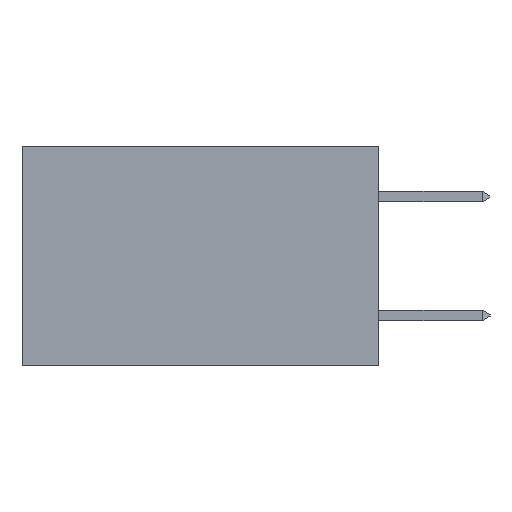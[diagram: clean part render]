
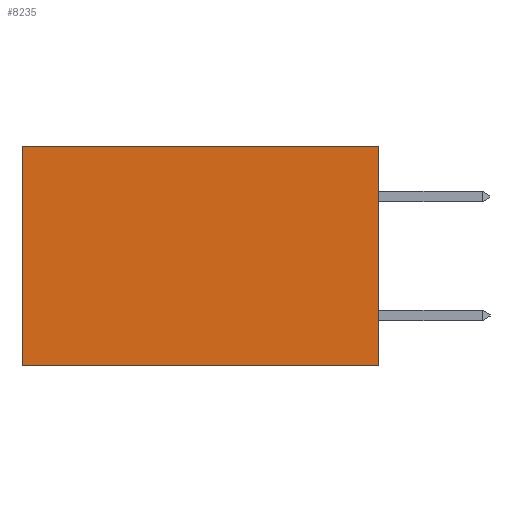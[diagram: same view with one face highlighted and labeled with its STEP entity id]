
A CAD part, left-side view. The second image highlights one B-rep face of the part: STEP entity #8235.
In plain terms, the highlighted planar face has unit normal (-1, 0, 0).
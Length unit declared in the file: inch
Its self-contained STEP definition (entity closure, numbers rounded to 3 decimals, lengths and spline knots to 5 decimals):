
#30 = DIRECTION ( 'NONE',  ( 1., 0., 0. ) ) ;
#205 = DIRECTION ( 'NONE',  ( 0., 0., -1. ) ) ;
#459 = VERTEX_POINT ( 'NONE', #10923 ) ;
#1226 = ORIENTED_EDGE ( 'NONE', *, *, #1270, .T. ) ;
#1270 = EDGE_CURVE ( 'NONE', #3533, #6409, #7976, .T. ) ;
#1271 = EDGE_CURVE ( 'NONE', #459, #3533, #5555, .T. ) ;
#1653 = ORIENTED_EDGE ( 'NONE', *, *, #2635, .F. ) ;
#2276 = CARTESIAN_POINT ( 'NONE',  ( 0.2615, 0.6, -0.37 ) ) ;
#2635 = EDGE_CURVE ( 'NONE', #5878, #6409, #6216, .T. ) ;
#3052 = VECTOR ( 'NONE', #205, 39.37008 ) ;
#3404 = EDGE_CURVE ( 'NONE', #459, #5878, #4467, .T. ) ;
#3533 = VERTEX_POINT ( 'NONE', #8649 ) ;
#4165 = VECTOR ( 'NONE', #7074, 39.37008 ) ;
#4459 = AXIS2_PLACEMENT_3D ( 'NONE', #5763, #30, #6706 ) ;
#4467 = LINE ( 'NONE', #4572, #4165 ) ;
#4572 = CARTESIAN_POINT ( 'NONE',  ( 0.2615, 0., -0.37 ) ) ;
#5555 = LINE ( 'NONE', #8586, #10123 ) ;
#5763 = CARTESIAN_POINT ( 'NONE',  ( 0.2615, 0., -0.37 ) ) ;
#5878 = VERTEX_POINT ( 'NONE', #11259 ) ;
#5910 = VECTOR ( 'NONE', #6240, 39.37008 ) ;
#6027 = ORIENTED_EDGE ( 'NONE', *, *, #3404, .F. ) ;
#6161 = CARTESIAN_POINT ( 'NONE',  ( 0.2615, 0., -0.37 ) ) ;
#6216 = LINE ( 'NONE', #6161, #5910 ) ;
#6240 = DIRECTION ( 'NONE',  ( 0., 1., 0. ) ) ;
#6409 = VERTEX_POINT ( 'NONE', #2276 ) ;
#6706 = DIRECTION ( 'NONE',  ( 0., 0., -1. ) ) ;
#7074 = DIRECTION ( 'NONE',  ( 0., 0., -1. ) ) ;
#7696 = EDGE_LOOP ( 'NONE', ( #1226, #1653, #6027, #8986 ) ) ;
#7871 = FACE_OUTER_BOUND ( 'NONE', #7696, .T. ) ;
#7976 = LINE ( 'NONE', #9638, #3052 ) ;
#8235 = ADVANCED_FACE ( 'NONE', ( #7871 ), #10306, .F. ) ;
#8365 = DIRECTION ( 'NONE',  ( 0., 1., 0. ) ) ;
#8586 = CARTESIAN_POINT ( 'NONE',  ( 0.2615, 0., 0. ) ) ;
#8649 = CARTESIAN_POINT ( 'NONE',  ( 0.2615, 0.6, 0. ) ) ;
#8986 = ORIENTED_EDGE ( 'NONE', *, *, #1271, .T. ) ;
#9638 = CARTESIAN_POINT ( 'NONE',  ( 0.2615, 0.6, -0.37 ) ) ;
#10123 = VECTOR ( 'NONE', #8365, 39.37008 ) ;
#10306 = PLANE ( 'NONE',  #4459 ) ;
#10923 = CARTESIAN_POINT ( 'NONE',  ( 0.2615, 0., 0. ) ) ;
#11259 = CARTESIAN_POINT ( 'NONE',  ( 0.2615, 0., -0.37 ) ) ;
